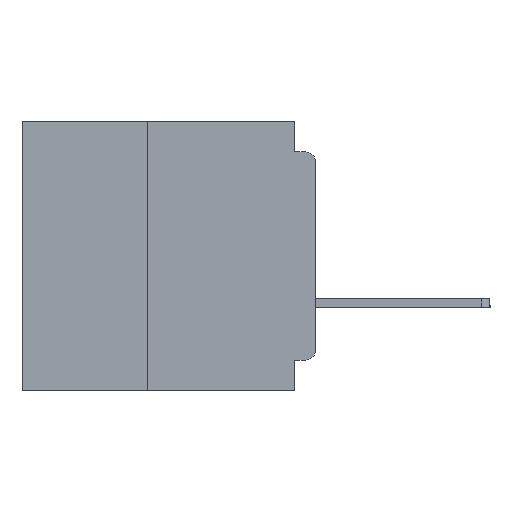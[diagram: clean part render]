
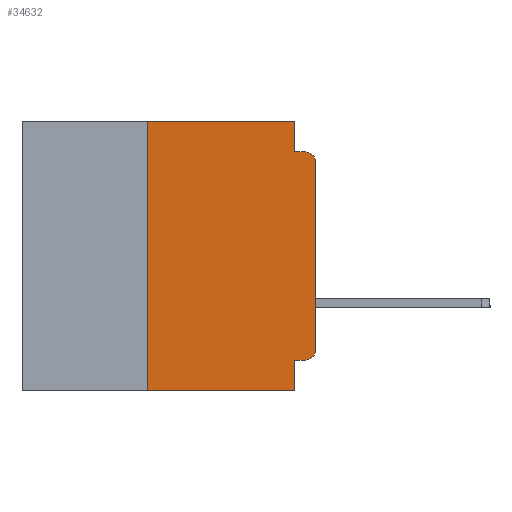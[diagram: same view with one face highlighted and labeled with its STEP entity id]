
A CAD part, left-side view. The second image highlights one B-rep face of the part: STEP entity #34632.
In plain terms, the highlighted planar face has unit normal (-1, 0, 0).
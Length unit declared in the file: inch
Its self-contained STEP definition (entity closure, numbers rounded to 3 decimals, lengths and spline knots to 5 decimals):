
#59 = VERTEX_POINT ( 'NONE', #48647 ) ;
#1326 = VERTEX_POINT ( 'NONE', #34423 ) ;
#1479 = VERTEX_POINT ( 'NONE', #18697 ) ;
#2127 = VERTEX_POINT ( 'NONE', #27502 ) ;
#3020 = LINE ( 'NONE', #40776, #22285 ) ;
#3689 = VERTEX_POINT ( 'NONE', #9977 ) ;
#4114 = CARTESIAN_POINT ( 'NONE',  ( 0., 0.015, -0.34 ) ) ;
#4427 = EDGE_CURVE ( 'NONE', #28351, #40730, #33840, .T. ) ;
#5201 = DIRECTION ( 'NONE',  ( 0., 0., -1. ) ) ;
#5900 = EDGE_CURVE ( 'NONE', #14476, #59, #13812, .T. ) ;
#6705 = VECTOR ( 'NONE', #38839, 39.37008 ) ;
#6981 = DIRECTION ( 'NONE',  ( 1., 0., 0. ) ) ;
#7580 = EDGE_CURVE ( 'NONE', #3689, #28351, #25730, .T. ) ;
#7982 = DIRECTION ( 'NONE',  ( 0., 0., -1. ) ) ;
#8429 = CIRCLE ( 'NONE', #9948, 0.015 ) ;
#8974 = VECTOR ( 'NONE', #45491, 39.37008 ) ;
#9237 = CARTESIAN_POINT ( 'NONE',  ( 0., 0.015, -0.355 ) ) ;
#9643 = CARTESIAN_POINT ( 'NONE',  ( 0., 0.031, -0.4 ) ) ;
#9948 = AXIS2_PLACEMENT_3D ( 'NONE', #4114, #31022, #7982 ) ;
#9977 = CARTESIAN_POINT ( 'NONE',  ( 0., 0.25, -0.4 ) ) ;
#11085 = ORIENTED_EDGE ( 'NONE', *, *, #44146, .F. ) ;
#12915 = CARTESIAN_POINT ( 'NONE',  ( 0., 0., -0.355 ) ) ;
#13616 = FACE_OUTER_BOUND ( 'NONE', #26726, .T. ) ;
#13812 = LINE ( 'NONE', #9643, #33052 ) ;
#14051 = ORIENTED_EDGE ( 'NONE', *, *, #39788, .F. ) ;
#14476 = VERTEX_POINT ( 'NONE', #17079 ) ;
#15882 = CARTESIAN_POINT ( 'NONE',  ( 0., 0., 0. ) ) ;
#16030 = CARTESIAN_POINT ( 'NONE',  ( 0., 0.015, -0.06 ) ) ;
#16585 = ORIENTED_EDGE ( 'NONE', *, *, #7580, .F. ) ;
#16870 = VECTOR ( 'NONE', #24916, 39.37008 ) ;
#17079 = CARTESIAN_POINT ( 'NONE',  ( 0., 0.031, -0.355 ) ) ;
#17363 = ORIENTED_EDGE ( 'NONE', *, *, #26011, .F. ) ;
#17381 = DIRECTION ( 'NONE',  ( 0., 0., -1. ) ) ;
#18450 = CARTESIAN_POINT ( 'NONE',  ( 0., 0.437, 0. ) ) ;
#18686 = LINE ( 'NONE', #12915, #47818 ) ;
#18697 = CARTESIAN_POINT ( 'NONE',  ( 0., 0., -0.06 ) ) ;
#19292 = LINE ( 'NONE', #21051, #16870 ) ;
#19729 = VERTEX_POINT ( 'NONE', #9237 ) ;
#19900 = DIRECTION ( 'NONE',  ( 0., 0., -1. ) ) ;
#21051 = CARTESIAN_POINT ( 'NONE',  ( 0., 0., -0.045 ) ) ;
#22024 = ORIENTED_EDGE ( 'NONE', *, *, #26095, .T. ) ;
#22285 = VECTOR ( 'NONE', #44524, 39.37008 ) ;
#22312 = AXIS2_PLACEMENT_3D ( 'NONE', #18450, #6981, #33888 ) ;
#22575 = CARTESIAN_POINT ( 'NONE',  ( 0., 0.437, 0. ) ) ;
#22853 = DIRECTION ( 'NONE',  ( 0., 0., 1. ) ) ;
#24373 = CARTESIAN_POINT ( 'NONE',  ( 0., 0.031, 0. ) ) ;
#24513 = DIRECTION ( 'NONE',  ( 0., 1., 0. ) ) ;
#24916 = DIRECTION ( 'NONE',  ( 0., -1., 0. ) ) ;
#25730 = LINE ( 'NONE', #49216, #44756 ) ;
#26011 = EDGE_CURVE ( 'NONE', #48873, #2127, #19292, .T. ) ;
#26095 = EDGE_CURVE ( 'NONE', #3689, #59, #3020, .T. ) ;
#26153 = PLANE ( 'NONE',  #22312 ) ;
#26305 = AXIS2_PLACEMENT_3D ( 'NONE', #16030, #42756, #19900 ) ;
#26726 = EDGE_LOOP ( 'NONE', ( #48821, #28739, #17363, #11085, #29382, #16585, #22024, #29336, #14051, #49095 ) ) ;
#26873 = EDGE_CURVE ( 'NONE', #19729, #1326, #8429, .T. ) ;
#27502 = CARTESIAN_POINT ( 'NONE',  ( 0., 0.015, -0.045 ) ) ;
#28351 = VERTEX_POINT ( 'NONE', #29366 ) ;
#28388 = LINE ( 'NONE', #15882, #6705 ) ;
#28739 = ORIENTED_EDGE ( 'NONE', *, *, #33576, .T. ) ;
#29336 = ORIENTED_EDGE ( 'NONE', *, *, #5900, .F. ) ;
#29366 = CARTESIAN_POINT ( 'NONE',  ( 0., 0.25, 0. ) ) ;
#29382 = ORIENTED_EDGE ( 'NONE', *, *, #4427, .F. ) ;
#31022 = DIRECTION ( 'NONE',  ( -1., 0., 0. ) ) ;
#31090 = EDGE_CURVE ( 'NONE', #1326, #1479, #28388, .T. ) ;
#31200 = CIRCLE ( 'NONE', #26305, 0.015 ) ;
#33052 = VECTOR ( 'NONE', #17381, 39.37008 ) ;
#33576 = EDGE_CURVE ( 'NONE', #1479, #2127, #31200, .T. ) ;
#33840 = LINE ( 'NONE', #22575, #8974 ) ;
#33888 = DIRECTION ( 'NONE',  ( 0., 0., -1. ) ) ;
#34423 = CARTESIAN_POINT ( 'NONE',  ( 0., 0., -0.34 ) ) ;
#34632 = ADVANCED_FACE ( 'NONE', ( #13616 ), #26153, .F. ) ;
#36192 = LINE ( 'NONE', #24373, #44999 ) ;
#38839 = DIRECTION ( 'NONE',  ( 0., 0., 1. ) ) ;
#39788 = EDGE_CURVE ( 'NONE', #19729, #14476, #18686, .T. ) ;
#40730 = VERTEX_POINT ( 'NONE', #49129 ) ;
#40776 = CARTESIAN_POINT ( 'NONE',  ( 0., 0.437, -0.4 ) ) ;
#41106 = CARTESIAN_POINT ( 'NONE',  ( 0., 0.031, -0.045 ) ) ;
#42756 = DIRECTION ( 'NONE',  ( -1., 0., 0. ) ) ;
#44146 = EDGE_CURVE ( 'NONE', #40730, #48873, #36192, .T. ) ;
#44524 = DIRECTION ( 'NONE',  ( 0., -1., 0. ) ) ;
#44756 = VECTOR ( 'NONE', #22853, 39.37008 ) ;
#44999 = VECTOR ( 'NONE', #5201, 39.37008 ) ;
#45491 = DIRECTION ( 'NONE',  ( 0., -1., 0. ) ) ;
#47818 = VECTOR ( 'NONE', #24513, 39.37008 ) ;
#48647 = CARTESIAN_POINT ( 'NONE',  ( 0., 0.031, -0.4 ) ) ;
#48821 = ORIENTED_EDGE ( 'NONE', *, *, #31090, .T. ) ;
#48873 = VERTEX_POINT ( 'NONE', #41106 ) ;
#49095 = ORIENTED_EDGE ( 'NONE', *, *, #26873, .T. ) ;
#49129 = CARTESIAN_POINT ( 'NONE',  ( 0., 0.031, 0. ) ) ;
#49216 = CARTESIAN_POINT ( 'NONE',  ( 0., 0.25, -0.4 ) ) ;
